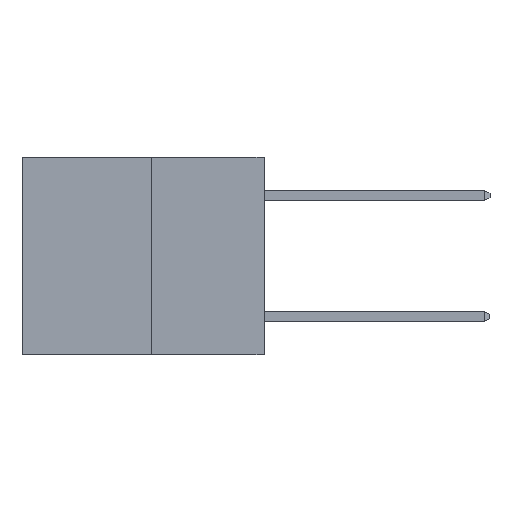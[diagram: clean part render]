
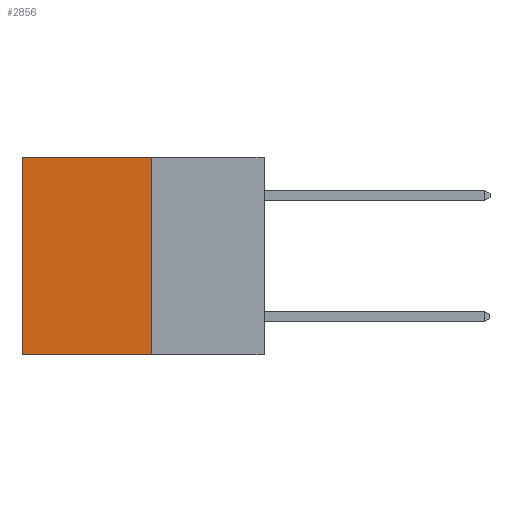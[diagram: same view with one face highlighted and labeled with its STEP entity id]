
A CAD part, left-side view. The second image highlights one B-rep face of the part: STEP entity #2856.
In plain terms, the highlighted planar face has unit normal (-1, 0, 0).
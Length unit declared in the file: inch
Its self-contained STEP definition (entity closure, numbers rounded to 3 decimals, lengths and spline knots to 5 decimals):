
#942 = LINE ( 'NONE', #8637, #8268 ) ;
#2134 = VERTEX_POINT ( 'NONE', #12842 ) ;
#2856 = ADVANCED_FACE ( 'NONE', ( #4006 ), #14678, .F. ) ;
#3182 = CARTESIAN_POINT ( 'NONE',  ( 0.3165, 0.28, -0.49 ) ) ;
#3756 = CARTESIAN_POINT ( 'NONE',  ( 0.3165, 0.28, -0.49 ) ) ;
#4006 = FACE_OUTER_BOUND ( 'NONE', #7189, .T. ) ;
#4378 = LINE ( 'NONE', #10184, #7401 ) ;
#4704 = ORIENTED_EDGE ( 'NONE', *, *, #5124, .F. ) ;
#5124 = EDGE_CURVE ( 'NONE', #11912, #7529, #13209, .T. ) ;
#5608 = LINE ( 'NONE', #6402, #7426 ) ;
#6402 = CARTESIAN_POINT ( 'NONE',  ( 0.3165, 0.28, -0.49 ) ) ;
#6711 = CARTESIAN_POINT ( 'NONE',  ( 0.3165, 0.28, -0.49 ) ) ;
#7189 = EDGE_LOOP ( 'NONE', ( #11310, #4704, #8848, #13943 ) ) ;
#7401 = VECTOR ( 'NONE', #16583, 39.37008 ) ;
#7426 = VECTOR ( 'NONE', #10141, 39.37008 ) ;
#7489 = DIRECTION ( 'NONE',  ( 0., 1., 0. ) ) ;
#7529 = VERTEX_POINT ( 'NONE', #10143 ) ;
#8268 = VECTOR ( 'NONE', #16283, 39.37008 ) ;
#8637 = CARTESIAN_POINT ( 'NONE',  ( 0.3165, 0.6, -0.49 ) ) ;
#8848 = ORIENTED_EDGE ( 'NONE', *, *, #14913, .F. ) ;
#9436 = DIRECTION ( 'NONE',  ( 0., 0., -1. ) ) ;
#9551 = VERTEX_POINT ( 'NONE', #16040 ) ;
#9793 = VECTOR ( 'NONE', #7489, 39.37008 ) ;
#9910 = AXIS2_PLACEMENT_3D ( 'NONE', #6711, #10617, #9436 ) ;
#10141 = DIRECTION ( 'NONE',  ( 0., 0., -1. ) ) ;
#10143 = CARTESIAN_POINT ( 'NONE',  ( 0.3165, 0.6, -0.49 ) ) ;
#10184 = CARTESIAN_POINT ( 'NONE',  ( 0.3165, 0.28, 0. ) ) ;
#10617 = DIRECTION ( 'NONE',  ( 1., 0., 0. ) ) ;
#11310 = ORIENTED_EDGE ( 'NONE', *, *, #13684, .T. ) ;
#11912 = VERTEX_POINT ( 'NONE', #3182 ) ;
#12555 = EDGE_CURVE ( 'NONE', #9551, #2134, #4378, .T. ) ;
#12842 = CARTESIAN_POINT ( 'NONE',  ( 0.3165, 0.6, 0. ) ) ;
#13209 = LINE ( 'NONE', #3756, #9793 ) ;
#13684 = EDGE_CURVE ( 'NONE', #2134, #7529, #942, .T. ) ;
#13943 = ORIENTED_EDGE ( 'NONE', *, *, #12555, .T. ) ;
#14678 = PLANE ( 'NONE',  #9910 ) ;
#14913 = EDGE_CURVE ( 'NONE', #9551, #11912, #5608, .T. ) ;
#16040 = CARTESIAN_POINT ( 'NONE',  ( 0.3165, 0.28, 0. ) ) ;
#16283 = DIRECTION ( 'NONE',  ( 0., 0., -1. ) ) ;
#16583 = DIRECTION ( 'NONE',  ( 0., 1., 0. ) ) ;
